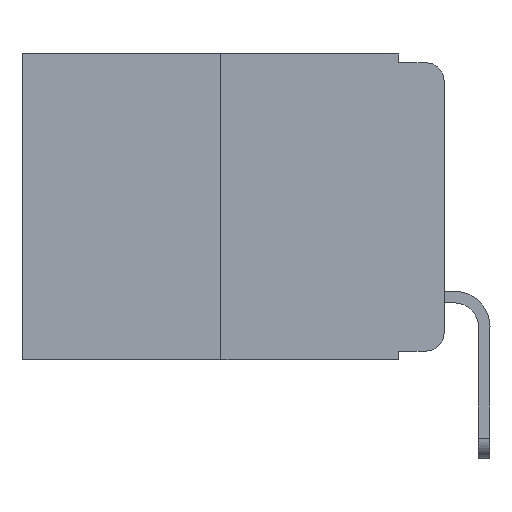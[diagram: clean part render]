
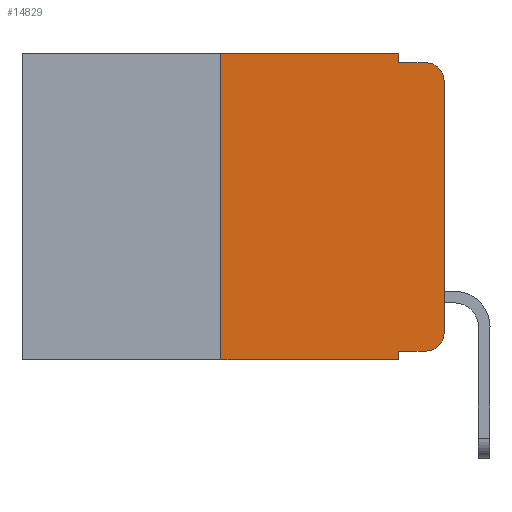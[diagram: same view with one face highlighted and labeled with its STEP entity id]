
A CAD part, left-side view. The second image highlights one B-rep face of the part: STEP entity #14829.
In plain terms, the highlighted planar face has unit normal (-1, 0, 0).
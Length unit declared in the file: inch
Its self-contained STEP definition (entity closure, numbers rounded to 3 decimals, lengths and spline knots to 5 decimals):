
#297 = ORIENTED_EDGE ( 'NONE', *, *, #16709, .T. ) ;
#305 = VECTOR ( 'NONE', #4595, 39.37008 ) ;
#403 = CARTESIAN_POINT ( 'NONE',  ( 0., 0.473, 0. ) ) ;
#480 = CARTESIAN_POINT ( 'NONE',  ( 0., 0.473, -0.343 ) ) ;
#778 = VERTEX_POINT ( 'NONE', #4729 ) ;
#786 = LINE ( 'NONE', #11993, #305 ) ;
#788 = CARTESIAN_POINT ( 'NONE',  ( 0., 0.051, -0.343 ) ) ;
#1678 = VERTEX_POINT ( 'NONE', #15425 ) ;
#2093 = CARTESIAN_POINT ( 'NONE',  ( 0., 0., 0. ) ) ;
#2647 = DIRECTION ( 'NONE',  ( 0., 0., -1. ) ) ;
#3054 = EDGE_CURVE ( 'NONE', #14828, #5212, #7790, .T. ) ;
#3742 = CARTESIAN_POINT ( 'NONE',  ( 0., 0.02, -0.01 ) ) ;
#3955 = CARTESIAN_POINT ( 'NONE',  ( 0., 0., -0.313 ) ) ;
#4082 = CIRCLE ( 'NONE', #14616, 0.02 ) ;
#4130 = LINE ( 'NONE', #2093, #18088 ) ;
#4254 = CARTESIAN_POINT ( 'NONE',  ( 0., 0.25, -0.343 ) ) ;
#4258 = DIRECTION ( 'NONE',  ( 0., 0., -1. ) ) ;
#4406 = VECTOR ( 'NONE', #7752, 39.37008 ) ;
#4425 = ORIENTED_EDGE ( 'NONE', *, *, #16342, .F. ) ;
#4595 = DIRECTION ( 'NONE',  ( 0., -1., 0. ) ) ;
#4729 = CARTESIAN_POINT ( 'NONE',  ( 0., 0.051, -0.333 ) ) ;
#4844 = VERTEX_POINT ( 'NONE', #14483 ) ;
#4972 = EDGE_CURVE ( 'NONE', #4844, #5212, #4082, .T. ) ;
#5084 = DIRECTION ( 'NONE',  ( 0., 0., -1. ) ) ;
#5212 = VERTEX_POINT ( 'NONE', #3742 ) ;
#5370 = ORIENTED_EDGE ( 'NONE', *, *, #17072, .F. ) ;
#5446 = VERTEX_POINT ( 'NONE', #8836 ) ;
#5845 = EDGE_CURVE ( 'NONE', #778, #5446, #786, .T. ) ;
#5984 = ORIENTED_EDGE ( 'NONE', *, *, #9619, .T. ) ;
#6299 = ORIENTED_EDGE ( 'NONE', *, *, #5845, .T. ) ;
#6558 = ORIENTED_EDGE ( 'NONE', *, *, #4972, .T. ) ;
#6689 = DIRECTION ( 'NONE',  ( 0., 0., 1. ) ) ;
#6751 = VECTOR ( 'NONE', #12889, 39.37008 ) ;
#7152 = CARTESIAN_POINT ( 'NONE',  ( 0., 0.051, -0.01 ) ) ;
#7221 = LINE ( 'NONE', #18410, #19085 ) ;
#7269 = PLANE ( 'NONE',  #16135 ) ;
#7474 = ORIENTED_EDGE ( 'NONE', *, *, #3054, .F. ) ;
#7752 = DIRECTION ( 'NONE',  ( 0., -1., 0. ) ) ;
#7790 = LINE ( 'NONE', #16074, #13828 ) ;
#8390 = VERTEX_POINT ( 'NONE', #4254 ) ;
#8807 = LINE ( 'NONE', #480, #4406 ) ;
#8836 = CARTESIAN_POINT ( 'NONE',  ( 0., 0.02, -0.333 ) ) ;
#9086 = VERTEX_POINT ( 'NONE', #3955 ) ;
#9619 = EDGE_CURVE ( 'NONE', #5446, #9086, #16217, .T. ) ;
#9922 = DIRECTION ( 'NONE',  ( -1., 0., 0. ) ) ;
#10122 = DIRECTION ( 'NONE',  ( 0., -1., 0. ) ) ;
#10134 = DIRECTION ( 'NONE',  ( -1., 0., 0. ) ) ;
#10551 = CARTESIAN_POINT ( 'NONE',  ( 0., 0.051, 0. ) ) ;
#10768 = VERTEX_POINT ( 'NONE', #13295 ) ;
#11195 = ORIENTED_EDGE ( 'NONE', *, *, #14464, .F. ) ;
#11335 = AXIS2_PLACEMENT_3D ( 'NONE', #15944, #9922, #2647 ) ;
#11919 = DIRECTION ( 'NONE',  ( 0., 0., -1. ) ) ;
#11993 = CARTESIAN_POINT ( 'NONE',  ( 0., 0.051, -0.333 ) ) ;
#12576 = FACE_OUTER_BOUND ( 'NONE', #14015, .T. ) ;
#12889 = DIRECTION ( 'NONE',  ( 0., 0., 1. ) ) ;
#13066 = LINE ( 'NONE', #403, #15861 ) ;
#13295 = CARTESIAN_POINT ( 'NONE',  ( 0., 0.25, 0. ) ) ;
#13345 = CARTESIAN_POINT ( 'NONE',  ( 0., 0.02, -0.03 ) ) ;
#13475 = ORIENTED_EDGE ( 'NONE', *, *, #18023, .T. ) ;
#13775 = DIRECTION ( 'NONE',  ( 0., -1., 0. ) ) ;
#13828 = VECTOR ( 'NONE', #10122, 39.37008 ) ;
#14015 = EDGE_LOOP ( 'NONE', ( #13475, #6558, #7474, #4425, #11195, #5370, #297, #14697, #6299, #5984 ) ) ;
#14464 = EDGE_CURVE ( 'NONE', #10768, #1678, #13066, .T. ) ;
#14483 = CARTESIAN_POINT ( 'NONE',  ( 0., 0., -0.03 ) ) ;
#14616 = AXIS2_PLACEMENT_3D ( 'NONE', #13345, #10134, #4258 ) ;
#14697 = ORIENTED_EDGE ( 'NONE', *, *, #19193, .F. ) ;
#14828 = VERTEX_POINT ( 'NONE', #7152 ) ;
#14829 = ADVANCED_FACE ( 'NONE', ( #12576 ), #7269, .F. ) ;
#15425 = CARTESIAN_POINT ( 'NONE',  ( 0., 0.051, 0. ) ) ;
#15861 = VECTOR ( 'NONE', #13775, 39.37008 ) ;
#15944 = CARTESIAN_POINT ( 'NONE',  ( 0., 0.02, -0.313 ) ) ;
#16074 = CARTESIAN_POINT ( 'NONE',  ( 0., 0.051, -0.01 ) ) ;
#16135 = AXIS2_PLACEMENT_3D ( 'NONE', #17678, #17618, #18980 ) ;
#16217 = CIRCLE ( 'NONE', #11335, 0.02 ) ;
#16342 = EDGE_CURVE ( 'NONE', #1678, #14828, #7221, .T. ) ;
#16709 = EDGE_CURVE ( 'NONE', #8390, #18388, #8807, .T. ) ;
#16880 = LINE ( 'NONE', #10551, #17807 ) ;
#17072 = EDGE_CURVE ( 'NONE', #8390, #10768, #18601, .T. ) ;
#17618 = DIRECTION ( 'NONE',  ( 1., 0., 0. ) ) ;
#17678 = CARTESIAN_POINT ( 'NONE',  ( 0., 0.473, 0. ) ) ;
#17807 = VECTOR ( 'NONE', #11919, 39.37008 ) ;
#18023 = EDGE_CURVE ( 'NONE', #9086, #4844, #4130, .T. ) ;
#18088 = VECTOR ( 'NONE', #6689, 39.37008 ) ;
#18388 = VERTEX_POINT ( 'NONE', #788 ) ;
#18410 = CARTESIAN_POINT ( 'NONE',  ( 0., 0.051, 0. ) ) ;
#18601 = LINE ( 'NONE', #18935, #6751 ) ;
#18935 = CARTESIAN_POINT ( 'NONE',  ( 0., 0.25, 0. ) ) ;
#18980 = DIRECTION ( 'NONE',  ( 0., 0., -1. ) ) ;
#19085 = VECTOR ( 'NONE', #5084, 39.37008 ) ;
#19193 = EDGE_CURVE ( 'NONE', #778, #18388, #16880, .T. ) ;
